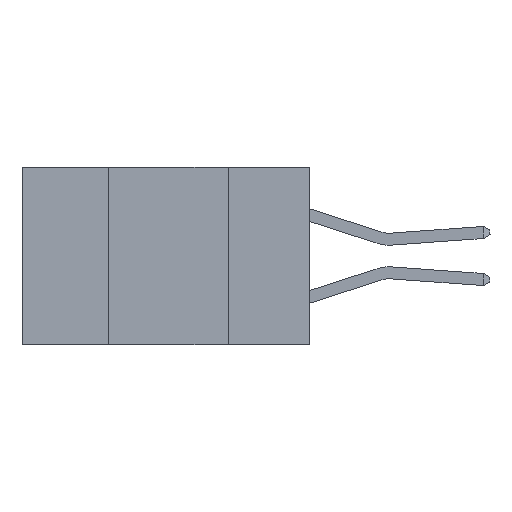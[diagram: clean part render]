
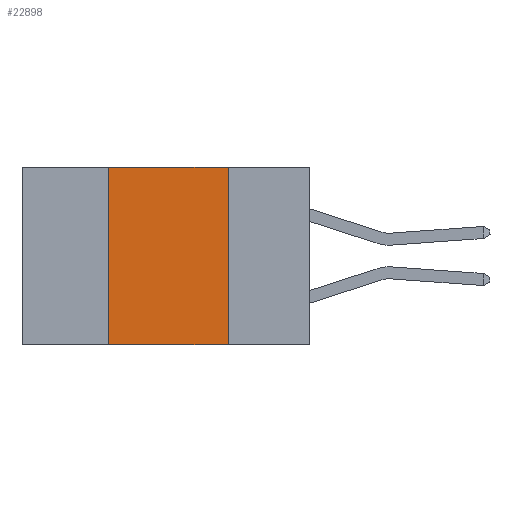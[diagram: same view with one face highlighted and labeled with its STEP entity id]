
A CAD part, left-side view. The second image highlights one B-rep face of the part: STEP entity #22898.
In plain terms, the highlighted planar face has unit normal (-1, 0, 0).
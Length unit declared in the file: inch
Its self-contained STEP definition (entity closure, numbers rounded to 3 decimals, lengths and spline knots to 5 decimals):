
#436 = LINE ( 'NONE', #2364, #26197 ) ;
#790 = CARTESIAN_POINT ( 'NONE',  ( 0., 0.42, 0. ) ) ;
#1383 = VERTEX_POINT ( 'NONE', #16165 ) ;
#1756 = CARTESIAN_POINT ( 'NONE',  ( 0., 0.6, 0. ) ) ;
#2178 = VECTOR ( 'NONE', #20243, 39.37008 ) ;
#2325 = LINE ( 'NONE', #790, #7148 ) ;
#2364 = CARTESIAN_POINT ( 'NONE',  ( 0., 0.17, 0. ) ) ;
#3892 = DIRECTION ( 'NONE',  ( 1., 0., 0. ) ) ;
#5198 = EDGE_CURVE ( 'NONE', #20383, #1383, #23260, .T. ) ;
#5257 = CARTESIAN_POINT ( 'NONE',  ( 0., 0.6, 0. ) ) ;
#5351 = DIRECTION ( 'NONE',  ( 0., -1., 0. ) ) ;
#6554 = FACE_OUTER_BOUND ( 'NONE', #26274, .T. ) ;
#7148 = VECTOR ( 'NONE', #13007, 39.37008 ) ;
#8012 = ORIENTED_EDGE ( 'NONE', *, *, #17463, .F. ) ;
#10164 = VERTEX_POINT ( 'NONE', #20736 ) ;
#10898 = AXIS2_PLACEMENT_3D ( 'NONE', #1756, #3892, #18186 ) ;
#11541 = ORIENTED_EDGE ( 'NONE', *, *, #23790, .F. ) ;
#13007 = DIRECTION ( 'NONE',  ( 0., 0., 1. ) ) ;
#14501 = EDGE_CURVE ( 'NONE', #21331, #10164, #26040, .T. ) ;
#14743 = ORIENTED_EDGE ( 'NONE', *, *, #5198, .T. ) ;
#16165 = CARTESIAN_POINT ( 'NONE',  ( 0., 0.17, -0.37 ) ) ;
#16779 = DIRECTION ( 'NONE',  ( 0., 0., -1. ) ) ;
#16896 = CARTESIAN_POINT ( 'NONE',  ( 0., 0.42, -0.37 ) ) ;
#17463 = EDGE_CURVE ( 'NONE', #20383, #21331, #2325, .T. ) ;
#18186 = DIRECTION ( 'NONE',  ( 0., 0., -1. ) ) ;
#19672 = CARTESIAN_POINT ( 'NONE',  ( 0., 0.6, -0.37 ) ) ;
#20243 = DIRECTION ( 'NONE',  ( 0., -1., 0. ) ) ;
#20383 = VERTEX_POINT ( 'NONE', #16896 ) ;
#20655 = VECTOR ( 'NONE', #5351, 39.37008 ) ;
#20736 = CARTESIAN_POINT ( 'NONE',  ( 0., 0.17, 0. ) ) ;
#21331 = VERTEX_POINT ( 'NONE', #26043 ) ;
#22898 = ADVANCED_FACE ( 'NONE', ( #6554 ), #26205, .F. ) ;
#23028 = ORIENTED_EDGE ( 'NONE', *, *, #14501, .F. ) ;
#23260 = LINE ( 'NONE', #19672, #2178 ) ;
#23790 = EDGE_CURVE ( 'NONE', #10164, #1383, #436, .T. ) ;
#26040 = LINE ( 'NONE', #5257, #20655 ) ;
#26043 = CARTESIAN_POINT ( 'NONE',  ( 0., 0.42, 0. ) ) ;
#26197 = VECTOR ( 'NONE', #16779, 39.37008 ) ;
#26205 = PLANE ( 'NONE',  #10898 ) ;
#26274 = EDGE_LOOP ( 'NONE', ( #11541, #23028, #8012, #14743 ) ) ;
